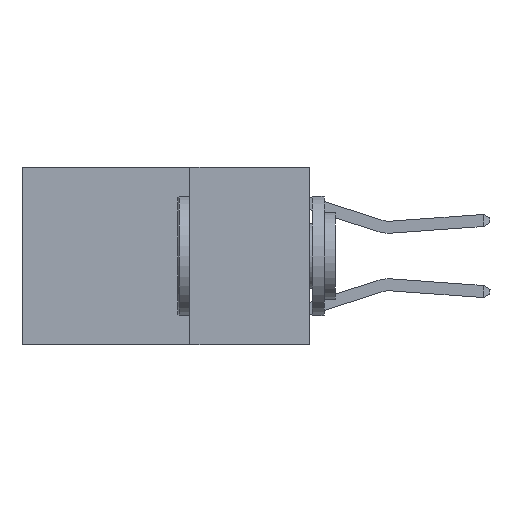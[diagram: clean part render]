
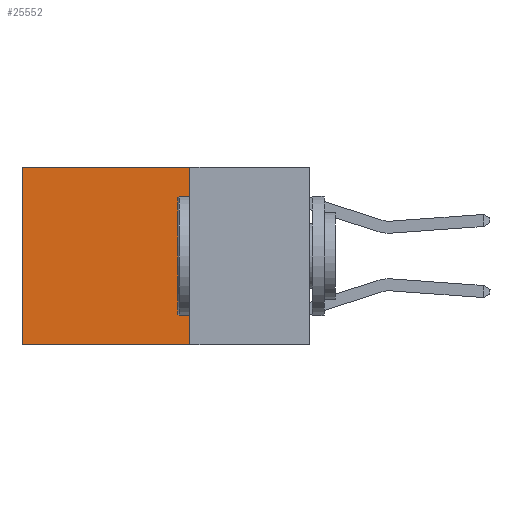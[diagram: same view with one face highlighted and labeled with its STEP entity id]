
A CAD part, left-side view. The second image highlights one B-rep face of the part: STEP entity #25552.
In plain terms, the highlighted planar face has unit normal (-1, 0, 0).
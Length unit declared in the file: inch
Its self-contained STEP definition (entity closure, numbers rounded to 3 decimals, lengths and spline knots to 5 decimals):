
#201 = DIRECTION ( 'NONE',  ( 0., 0., -1. ) ) ;
#273 = ORIENTED_EDGE ( 'NONE', *, *, #22678, .F. ) ;
#1334 = DIRECTION ( 'NONE',  ( 0., 0., -1. ) ) ;
#1682 = CARTESIAN_POINT ( 'NONE',  ( 0.2625, 0.25, 0. ) ) ;
#2054 = LINE ( 'NONE', #20218, #11866 ) ;
#2128 = CARTESIAN_POINT ( 'NONE',  ( 0.2625, 0.25, 0. ) ) ;
#3497 = DIRECTION ( 'NONE',  ( 0., 1., 0. ) ) ;
#3582 = ORIENTED_EDGE ( 'NONE', *, *, #28191, .T. ) ;
#4545 = DIRECTION ( 'NONE',  ( 0., 1., 0. ) ) ;
#7615 = VECTOR ( 'NONE', #10874, 39.37008 ) ;
#9170 = CARTESIAN_POINT ( 'NONE',  ( 0.2625, 0.6, 0. ) ) ;
#10874 = DIRECTION ( 'NONE',  ( 0., 0., -1. ) ) ;
#11725 = CARTESIAN_POINT ( 'NONE',  ( 0.2625, 0.25, 0. ) ) ;
#11866 = VECTOR ( 'NONE', #1334, 39.37008 ) ;
#14378 = CARTESIAN_POINT ( 'NONE',  ( 0.2625, 0.25, 0. ) ) ;
#14735 = CARTESIAN_POINT ( 'NONE',  ( 0.2625, 0.25, -0.37 ) ) ;
#14965 = CARTESIAN_POINT ( 'NONE',  ( 0.2625, 0.25, -0.37 ) ) ;
#16566 = LINE ( 'NONE', #14965, #18058 ) ;
#16726 = ORIENTED_EDGE ( 'NONE', *, *, #26208, .T. ) ;
#17498 = ORIENTED_EDGE ( 'NONE', *, *, #26607, .F. ) ;
#18058 = VECTOR ( 'NONE', #3497, 39.37008 ) ;
#18633 = FACE_OUTER_BOUND ( 'NONE', #23112, .T. ) ;
#19502 = VERTEX_POINT ( 'NONE', #11725 ) ;
#20218 = CARTESIAN_POINT ( 'NONE',  ( 0.2625, 0.6, 0. ) ) ;
#20864 = CARTESIAN_POINT ( 'NONE',  ( 0.2625, 0.6, -0.37 ) ) ;
#21273 = AXIS2_PLACEMENT_3D ( 'NONE', #14378, #21523, #201 ) ;
#21523 = DIRECTION ( 'NONE',  ( 1., 0., 0. ) ) ;
#21542 = VECTOR ( 'NONE', #4545, 39.37008 ) ;
#22678 = EDGE_CURVE ( 'NONE', #26517, #23323, #16566, .T. ) ;
#23112 = EDGE_LOOP ( 'NONE', ( #3582, #273, #17498, #16726 ) ) ;
#23323 = VERTEX_POINT ( 'NONE', #20864 ) ;
#25552 = ADVANCED_FACE ( 'NONE', ( #18633 ), #28213, .F. ) ;
#26208 = EDGE_CURVE ( 'NONE', #19502, #26857, #27808, .T. ) ;
#26517 = VERTEX_POINT ( 'NONE', #14735 ) ;
#26607 = EDGE_CURVE ( 'NONE', #19502, #26517, #27779, .T. ) ;
#26857 = VERTEX_POINT ( 'NONE', #9170 ) ;
#27779 = LINE ( 'NONE', #1682, #7615 ) ;
#27808 = LINE ( 'NONE', #2128, #21542 ) ;
#28191 = EDGE_CURVE ( 'NONE', #26857, #23323, #2054, .T. ) ;
#28213 = PLANE ( 'NONE',  #21273 ) ;
